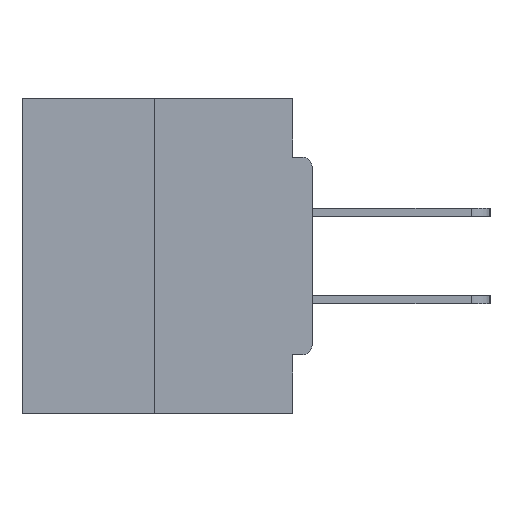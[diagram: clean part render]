
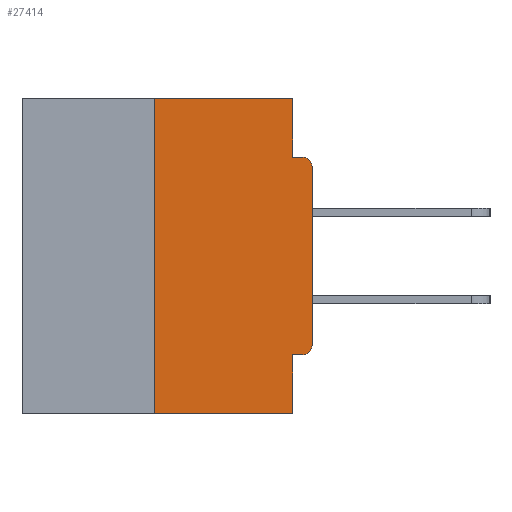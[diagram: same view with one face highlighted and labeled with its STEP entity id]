
A CAD part, left-side view. The second image highlights one B-rep face of the part: STEP entity #27414.
In plain terms, the highlighted planar face has unit normal (-1, 0, 0).
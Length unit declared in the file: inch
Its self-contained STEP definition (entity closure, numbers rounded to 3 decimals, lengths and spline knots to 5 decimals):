
#145 = LINE ( 'NONE', #8968, #16985 ) ;
#339 = EDGE_CURVE ( 'NONE', #8416, #9279, #3234, .T. ) ;
#1108 = ORIENTED_EDGE ( 'NONE', *, *, #19115, .T. ) ;
#1529 = ORIENTED_EDGE ( 'NONE', *, *, #26128, .T. ) ;
#2102 = CARTESIAN_POINT ( 'NONE',  ( 0., 0., 0. ) ) ;
#2250 = VERTEX_POINT ( 'NONE', #12615 ) ;
#2582 = CARTESIAN_POINT ( 'NONE',  ( 0., 0.25, 0. ) ) ;
#2961 = AXIS2_PLACEMENT_3D ( 'NONE', #9851, #9619, #20035 ) ;
#3158 = LINE ( 'NONE', #5913, #4419 ) ;
#3189 = ORIENTED_EDGE ( 'NONE', *, *, #33144, .T. ) ;
#3234 = LINE ( 'NONE', #15057, #25342 ) ;
#3374 = CARTESIAN_POINT ( 'NONE',  ( 0., 0.031, 0. ) ) ;
#3607 = EDGE_CURVE ( 'NONE', #6984, #8416, #12264, .T. ) ;
#4143 = VERTEX_POINT ( 'NONE', #5026 ) ;
#4203 = ORIENTED_EDGE ( 'NONE', *, *, #21689, .F. ) ;
#4419 = VECTOR ( 'NONE', #13323, 39.37008 ) ;
#5026 = CARTESIAN_POINT ( 'NONE',  ( 0., 0., -0.3915 ) ) ;
#5381 = ORIENTED_EDGE ( 'NONE', *, *, #13380, .F. ) ;
#5411 = CARTESIAN_POINT ( 'NONE',  ( 0., 0.25, -0.5 ) ) ;
#5439 = AXIS2_PLACEMENT_3D ( 'NONE', #6617, #27138, #8859 ) ;
#5913 = CARTESIAN_POINT ( 'NONE',  ( 0., 0., -0.0935 ) ) ;
#6617 = CARTESIAN_POINT ( 'NONE',  ( 0., 0.46, 0. ) ) ;
#6984 = VERTEX_POINT ( 'NONE', #5411 ) ;
#7254 = DIRECTION ( 'NONE',  ( 0., 0., 1. ) ) ;
#7537 = VECTOR ( 'NONE', #7254, 39.37008 ) ;
#8189 = VECTOR ( 'NONE', #27993, 39.37008 ) ;
#8416 = VERTEX_POINT ( 'NONE', #2582 ) ;
#8859 = DIRECTION ( 'NONE',  ( 0., 0., -1. ) ) ;
#8968 = CARTESIAN_POINT ( 'NONE',  ( 0., 0., -0.4065 ) ) ;
#9279 = VERTEX_POINT ( 'NONE', #3374 ) ;
#9619 = DIRECTION ( 'NONE',  ( -1., 0., 0. ) ) ;
#9851 = CARTESIAN_POINT ( 'NONE',  ( 0., 0.015, -0.3915 ) ) ;
#10708 = AXIS2_PLACEMENT_3D ( 'NONE', #18661, #23867, #26445 ) ;
#10937 = ORIENTED_EDGE ( 'NONE', *, *, #3607, .F. ) ;
#11194 = DIRECTION ( 'NONE',  ( 0., 0., -1. ) ) ;
#11883 = VECTOR ( 'NONE', #20051, 39.37008 ) ;
#12264 = LINE ( 'NONE', #28716, #20226 ) ;
#12431 = EDGE_CURVE ( 'NONE', #22186, #19211, #3158, .T. ) ;
#12615 = CARTESIAN_POINT ( 'NONE',  ( 0., 0., -0.1085 ) ) ;
#12808 = CARTESIAN_POINT ( 'NONE',  ( 0., 0.031, -0.4065 ) ) ;
#13141 = ORIENTED_EDGE ( 'NONE', *, *, #20906, .F. ) ;
#13323 = DIRECTION ( 'NONE',  ( 0., -1., 0. ) ) ;
#13380 = EDGE_CURVE ( 'NONE', #27182, #24461, #29572, .T. ) ;
#13531 = VECTOR ( 'NONE', #11194, 39.37008 ) ;
#13890 = PLANE ( 'NONE',  #5439 ) ;
#14600 = FACE_OUTER_BOUND ( 'NONE', #30109, .T. ) ;
#14902 = VERTEX_POINT ( 'NONE', #26361 ) ;
#15039 = CIRCLE ( 'NONE', #2961, 0.015 ) ;
#15057 = CARTESIAN_POINT ( 'NONE',  ( 0., 0.46, 0. ) ) ;
#15816 = CARTESIAN_POINT ( 'NONE',  ( 0., 0.031, -0.0935 ) ) ;
#16331 = LINE ( 'NONE', #2102, #7537 ) ;
#16560 = LINE ( 'NONE', #25325, #8189 ) ;
#16985 = VECTOR ( 'NONE', #26817, 39.37008 ) ;
#18587 = DIRECTION ( 'NONE',  ( 0., 0., 1. ) ) ;
#18661 = CARTESIAN_POINT ( 'NONE',  ( 0., 0.015, -0.1085 ) ) ;
#19115 = EDGE_CURVE ( 'NONE', #4143, #2250, #16331, .T. ) ;
#19211 = VERTEX_POINT ( 'NONE', #32900 ) ;
#19539 = CIRCLE ( 'NONE', #10708, 0.015 ) ;
#20035 = DIRECTION ( 'NONE',  ( 0., 0., -1. ) ) ;
#20051 = DIRECTION ( 'NONE',  ( 0., 0., -1. ) ) ;
#20226 = VECTOR ( 'NONE', #18587, 39.37008 ) ;
#20230 = DIRECTION ( 'NONE',  ( 0., -1., 0. ) ) ;
#20350 = CARTESIAN_POINT ( 'NONE',  ( 0., 0.031, -0.5 ) ) ;
#20906 = EDGE_CURVE ( 'NONE', #9279, #22186, #32302, .T. ) ;
#21689 = EDGE_CURVE ( 'NONE', #14902, #27182, #145, .T. ) ;
#22140 = EDGE_CURVE ( 'NONE', #6984, #24461, #16560, .T. ) ;
#22186 = VERTEX_POINT ( 'NONE', #15816 ) ;
#23867 = DIRECTION ( 'NONE',  ( -1., 0., 0. ) ) ;
#24461 = VERTEX_POINT ( 'NONE', #20350 ) ;
#25325 = CARTESIAN_POINT ( 'NONE',  ( 0., 0.46, -0.5 ) ) ;
#25342 = VECTOR ( 'NONE', #20230, 39.37008 ) ;
#26128 = EDGE_CURVE ( 'NONE', #2250, #19211, #19539, .T. ) ;
#26348 = CARTESIAN_POINT ( 'NONE',  ( 0., 0.031, -0.5 ) ) ;
#26361 = CARTESIAN_POINT ( 'NONE',  ( 0., 0.015, -0.4065 ) ) ;
#26445 = DIRECTION ( 'NONE',  ( 0., 0., -1. ) ) ;
#26560 = ORIENTED_EDGE ( 'NONE', *, *, #22140, .T. ) ;
#26817 = DIRECTION ( 'NONE',  ( 0., 1., 0. ) ) ;
#27138 = DIRECTION ( 'NONE',  ( 1., 0., 0. ) ) ;
#27182 = VERTEX_POINT ( 'NONE', #12808 ) ;
#27414 = ADVANCED_FACE ( 'NONE', ( #14600 ), #13890, .F. ) ;
#27993 = DIRECTION ( 'NONE',  ( 0., -1., 0. ) ) ;
#28716 = CARTESIAN_POINT ( 'NONE',  ( 0., 0.25, 0. ) ) ;
#29097 = ORIENTED_EDGE ( 'NONE', *, *, #12431, .F. ) ;
#29572 = LINE ( 'NONE', #26348, #13531 ) ;
#30109 = EDGE_LOOP ( 'NONE', ( #30481, #10937, #26560, #5381, #4203, #3189, #1108, #1529, #29097, #13141 ) ) ;
#30455 = CARTESIAN_POINT ( 'NONE',  ( 0., 0.031, 0. ) ) ;
#30481 = ORIENTED_EDGE ( 'NONE', *, *, #339, .F. ) ;
#32302 = LINE ( 'NONE', #30455, #11883 ) ;
#32900 = CARTESIAN_POINT ( 'NONE',  ( 0., 0.015, -0.0935 ) ) ;
#33144 = EDGE_CURVE ( 'NONE', #14902, #4143, #15039, .T. ) ;
